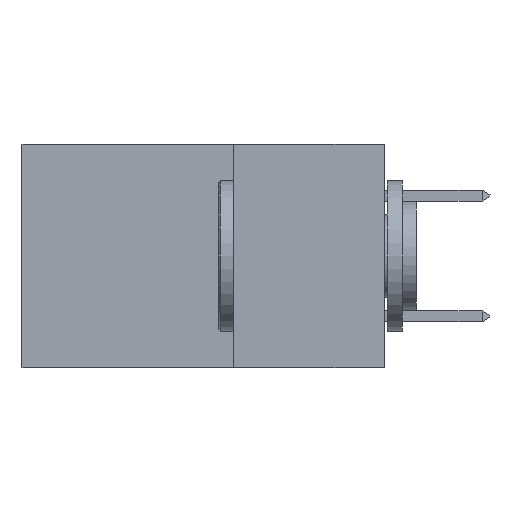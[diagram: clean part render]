
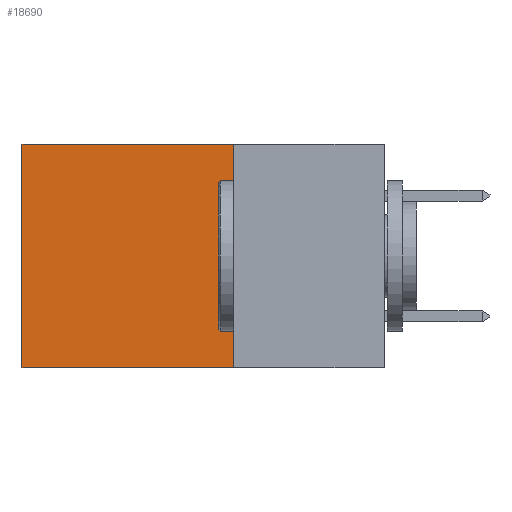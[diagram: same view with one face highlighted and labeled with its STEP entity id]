
A CAD part, left-side view. The second image highlights one B-rep face of the part: STEP entity #18690.
In plain terms, the highlighted planar face has unit normal (-1, 0, 0).
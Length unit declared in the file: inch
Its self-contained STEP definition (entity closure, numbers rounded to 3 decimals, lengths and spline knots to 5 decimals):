
#1376 = CARTESIAN_POINT ( 'NONE',  ( 0.2875, 0.6, -0.37 ) ) ;
#1678 = LINE ( 'NONE', #13891, #18857 ) ;
#1929 = DIRECTION ( 'NONE',  ( 0., 0., -1. ) ) ;
#1954 = VECTOR ( 'NONE', #11607, 39.37008 ) ;
#2755 = EDGE_CURVE ( 'NONE', #14756, #12212, #20478, .T. ) ;
#3708 = DIRECTION ( 'NONE',  ( 0., 0., -1. ) ) ;
#4242 = EDGE_CURVE ( 'NONE', #20810, #24126, #20421, .T. ) ;
#6697 = VECTOR ( 'NONE', #16790, 39.37008 ) ;
#6843 = ORIENTED_EDGE ( 'NONE', *, *, #2755, .F. ) ;
#9624 = CARTESIAN_POINT ( 'NONE',  ( 0.2875, 0.25, 0. ) ) ;
#9651 = CARTESIAN_POINT ( 'NONE',  ( 0.2875, 0.25, 0. ) ) ;
#9993 = EDGE_LOOP ( 'NONE', ( #10032, #6843, #18014, #15641 ) ) ;
#10032 = ORIENTED_EDGE ( 'NONE', *, *, #11887, .T. ) ;
#10714 = FACE_OUTER_BOUND ( 'NONE', #9993, .T. ) ;
#11607 = DIRECTION ( 'NONE',  ( 0., 0., -1. ) ) ;
#11887 = EDGE_CURVE ( 'NONE', #24126, #12212, #1678, .T. ) ;
#12212 = VERTEX_POINT ( 'NONE', #1376 ) ;
#13670 = DIRECTION ( 'NONE',  ( 1., 0., 0. ) ) ;
#13891 = CARTESIAN_POINT ( 'NONE',  ( 0.2875, 0.6, 0. ) ) ;
#14756 = VERTEX_POINT ( 'NONE', #15438 ) ;
#15112 = CARTESIAN_POINT ( 'NONE',  ( 0.2875, 0.25, 0. ) ) ;
#15438 = CARTESIAN_POINT ( 'NONE',  ( 0.2875, 0.25, -0.37 ) ) ;
#15641 = ORIENTED_EDGE ( 'NONE', *, *, #4242, .T. ) ;
#16325 = LINE ( 'NONE', #9651, #1954 ) ;
#16790 = DIRECTION ( 'NONE',  ( 0., 1., 0. ) ) ;
#17415 = AXIS2_PLACEMENT_3D ( 'NONE', #9624, #13670, #3708 ) ;
#17817 = EDGE_CURVE ( 'NONE', #20810, #14756, #16325, .T. ) ;
#18014 = ORIENTED_EDGE ( 'NONE', *, *, #17817, .F. ) ;
#18690 = ADVANCED_FACE ( 'NONE', ( #10714 ), #21469, .F. ) ;
#18857 = VECTOR ( 'NONE', #1929, 39.37008 ) ;
#19506 = VECTOR ( 'NONE', #21090, 39.37008 ) ;
#20215 = CARTESIAN_POINT ( 'NONE',  ( 0.2875, 0.6, 0. ) ) ;
#20421 = LINE ( 'NONE', #15112, #19506 ) ;
#20478 = LINE ( 'NONE', #20822, #6697 ) ;
#20810 = VERTEX_POINT ( 'NONE', #25940 ) ;
#20822 = CARTESIAN_POINT ( 'NONE',  ( 0.2875, 0.25, -0.37 ) ) ;
#21090 = DIRECTION ( 'NONE',  ( 0., 1., 0. ) ) ;
#21469 = PLANE ( 'NONE',  #17415 ) ;
#24126 = VERTEX_POINT ( 'NONE', #20215 ) ;
#25940 = CARTESIAN_POINT ( 'NONE',  ( 0.2875, 0.25, 0. ) ) ;
